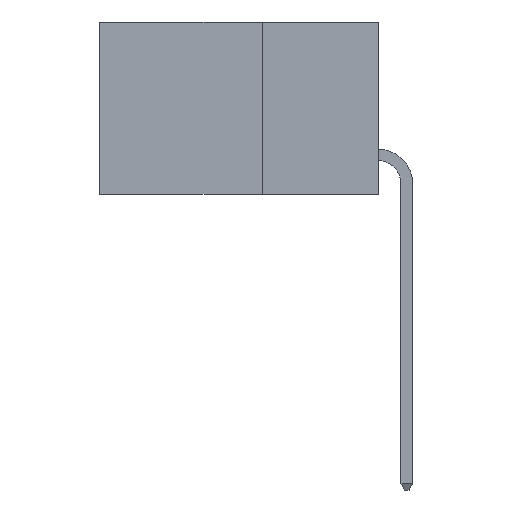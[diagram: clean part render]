
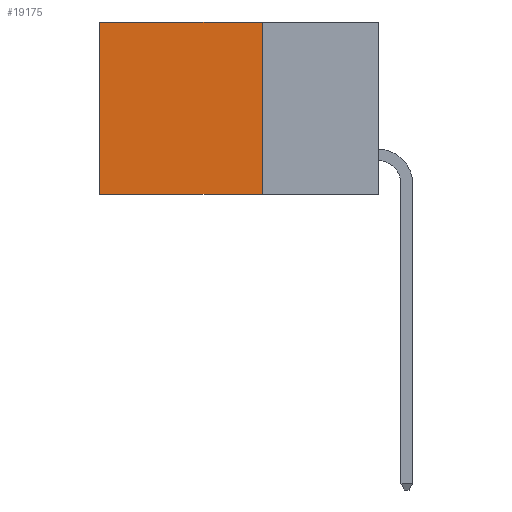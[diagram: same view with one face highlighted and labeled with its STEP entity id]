
A CAD part, left-side view. The second image highlights one B-rep face of the part: STEP entity #19175.
In plain terms, the highlighted planar face has unit normal (-1, 0, 0).
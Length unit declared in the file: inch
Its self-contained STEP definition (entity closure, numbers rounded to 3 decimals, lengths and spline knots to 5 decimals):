
#706 = LINE ( 'NONE', #21442, #19192 ) ;
#1271 = ORIENTED_EDGE ( 'NONE', *, *, #21873, .F. ) ;
#1336 = CARTESIAN_POINT ( 'NONE',  ( 0.2615, 0.25, -0.37 ) ) ;
#1695 = VERTEX_POINT ( 'NONE', #1747 ) ;
#1747 = CARTESIAN_POINT ( 'NONE',  ( 0.2615, 0.25, -0.37 ) ) ;
#3495 = EDGE_CURVE ( 'NONE', #1695, #19968, #11933, .T. ) ;
#3646 = CARTESIAN_POINT ( 'NONE',  ( 0.2615, 0.25, -0.37 ) ) ;
#4256 = CARTESIAN_POINT ( 'NONE',  ( 0.2615, 0.6, -0.37 ) ) ;
#4777 = ORIENTED_EDGE ( 'NONE', *, *, #21694, .T. ) ;
#5522 = DIRECTION ( 'NONE',  ( 0., 0., -1. ) ) ;
#6931 = VECTOR ( 'NONE', #22409, 39.37008 ) ;
#6974 = DIRECTION ( 'NONE',  ( 0., 0., -1. ) ) ;
#7410 = CARTESIAN_POINT ( 'NONE',  ( 0.2615, 0.25, 0. ) ) ;
#7978 = VECTOR ( 'NONE', #6974, 39.37008 ) ;
#11933 = LINE ( 'NONE', #23208, #6931 ) ;
#12407 = ORIENTED_EDGE ( 'NONE', *, *, #12694, .T. ) ;
#12694 = EDGE_CURVE ( 'NONE', #20596, #19968, #706, .T. ) ;
#12942 = LINE ( 'NONE', #1336, #7978 ) ;
#13004 = PLANE ( 'NONE',  #17193 ) ;
#14387 = DIRECTION ( 'NONE',  ( 0., 0., -1. ) ) ;
#16627 = CARTESIAN_POINT ( 'NONE',  ( 0.2615, 0.25, 0. ) ) ;
#16711 = DIRECTION ( 'NONE',  ( 1., 0., 0. ) ) ;
#17193 = AXIS2_PLACEMENT_3D ( 'NONE', #3646, #16711, #5522 ) ;
#17362 = CARTESIAN_POINT ( 'NONE',  ( 0.2615, 0.6, 0. ) ) ;
#18469 = DIRECTION ( 'NONE',  ( 0., 1., 0. ) ) ;
#19094 = EDGE_LOOP ( 'NONE', ( #12407, #22500, #1271, #4777 ) ) ;
#19175 = ADVANCED_FACE ( 'NONE', ( #22789 ), #13004, .F. ) ;
#19192 = VECTOR ( 'NONE', #14387, 39.37008 ) ;
#19220 = VERTEX_POINT ( 'NONE', #16627 ) ;
#19968 = VERTEX_POINT ( 'NONE', #4256 ) ;
#20596 = VERTEX_POINT ( 'NONE', #17362 ) ;
#21442 = CARTESIAN_POINT ( 'NONE',  ( 0.2615, 0.6, -0.37 ) ) ;
#21605 = VECTOR ( 'NONE', #18469, 39.37008 ) ;
#21694 = EDGE_CURVE ( 'NONE', #19220, #20596, #22140, .T. ) ;
#21873 = EDGE_CURVE ( 'NONE', #19220, #1695, #12942, .T. ) ;
#22140 = LINE ( 'NONE', #7410, #21605 ) ;
#22409 = DIRECTION ( 'NONE',  ( 0., 1., 0. ) ) ;
#22500 = ORIENTED_EDGE ( 'NONE', *, *, #3495, .F. ) ;
#22789 = FACE_OUTER_BOUND ( 'NONE', #19094, .T. ) ;
#23208 = CARTESIAN_POINT ( 'NONE',  ( 0.2615, 0.25, -0.37 ) ) ;
